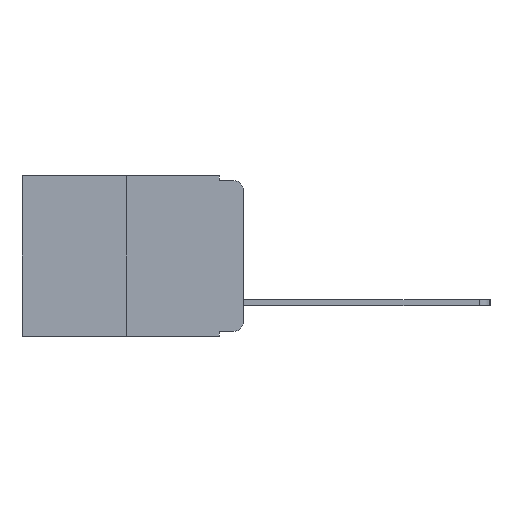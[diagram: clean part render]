
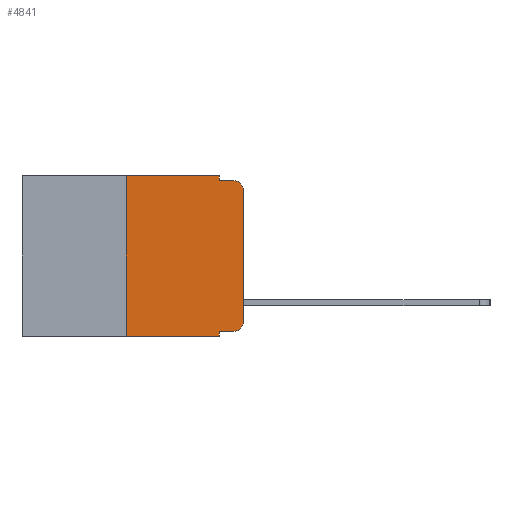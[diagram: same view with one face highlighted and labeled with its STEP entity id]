
A CAD part, left-side view. The second image highlights one B-rep face of the part: STEP entity #4841.
In plain terms, the highlighted planar face has unit normal (-1, 0, 0).
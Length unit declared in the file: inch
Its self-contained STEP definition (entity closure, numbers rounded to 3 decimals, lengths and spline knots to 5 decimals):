
#115 = ORIENTED_EDGE ( 'NONE', *, *, #9073, .F. ) ;
#141 = DIRECTION ( 'NONE',  ( 0., -1., 0. ) ) ;
#183 = CARTESIAN_POINT ( 'NONE',  ( 0., 0.02, -0.333 ) ) ;
#199 = DIRECTION ( 'NONE',  ( -1., 0., 0. ) ) ;
#259 = DIRECTION ( 'NONE',  ( 0., -1., 0. ) ) ;
#313 = VECTOR ( 'NONE', #8239, 39.37008 ) ;
#364 = VECTOR ( 'NONE', #259, 39.37008 ) ;
#525 = CARTESIAN_POINT ( 'NONE',  ( 0., 0.25, 0. ) ) ;
#972 = VECTOR ( 'NONE', #3164, 39.37008 ) ;
#1045 = VERTEX_POINT ( 'NONE', #7427 ) ;
#1091 = VERTEX_POINT ( 'NONE', #3987 ) ;
#1129 = VECTOR ( 'NONE', #141, 39.37008 ) ;
#1151 = DIRECTION ( 'NONE',  ( 0., 0., -1. ) ) ;
#1153 = LINE ( 'NONE', #5002, #7316 ) ;
#1173 = DIRECTION ( 'NONE',  ( 0., 0., 1. ) ) ;
#1389 = CARTESIAN_POINT ( 'NONE',  ( 0., 0.02, -0.313 ) ) ;
#1415 = LINE ( 'NONE', #10607, #1129 ) ;
#1475 = EDGE_CURVE ( 'NONE', #5974, #2383, #7640, .T. ) ;
#1546 = CARTESIAN_POINT ( 'NONE',  ( 0., 0.051, 0. ) ) ;
#1786 = VERTEX_POINT ( 'NONE', #6154 ) ;
#1915 = DIRECTION ( 'NONE',  ( 0., -1., 0. ) ) ;
#2142 = DIRECTION ( 'NONE',  ( 1., 0., 0. ) ) ;
#2383 = VERTEX_POINT ( 'NONE', #1546 ) ;
#2727 = CARTESIAN_POINT ( 'NONE',  ( 0., 0.051, -0.01 ) ) ;
#2735 = ORIENTED_EDGE ( 'NONE', *, *, #7925, .T. ) ;
#2810 = CARTESIAN_POINT ( 'NONE',  ( 0., 0.051, -0.01 ) ) ;
#2993 = VERTEX_POINT ( 'NONE', #4615 ) ;
#3016 = EDGE_CURVE ( 'NONE', #1786, #1045, #1415, .T. ) ;
#3032 = EDGE_CURVE ( 'NONE', #6423, #1091, #10123, .T. ) ;
#3164 = DIRECTION ( 'NONE',  ( 0., 0., 1. ) ) ;
#3453 = ORIENTED_EDGE ( 'NONE', *, *, #6531, .F. ) ;
#3987 = CARTESIAN_POINT ( 'NONE',  ( 0., 0.02, -0.01 ) ) ;
#4175 = AXIS2_PLACEMENT_3D ( 'NONE', #5494, #199, #6338 ) ;
#4245 = EDGE_CURVE ( 'NONE', #1786, #5974, #5395, .T. ) ;
#4615 = CARTESIAN_POINT ( 'NONE',  ( 0., 0., -0.313 ) ) ;
#4723 = CARTESIAN_POINT ( 'NONE',  ( 0., 0., 0. ) ) ;
#4762 = CARTESIAN_POINT ( 'NONE',  ( 0., 0.051, 0. ) ) ;
#4841 = ADVANCED_FACE ( 'NONE', ( #8622 ), #7584, .F. ) ;
#4946 = ORIENTED_EDGE ( 'NONE', *, *, #8287, .T. ) ;
#5002 = CARTESIAN_POINT ( 'NONE',  ( 0., 0.051, -0.333 ) ) ;
#5014 = EDGE_CURVE ( 'NONE', #6117, #2993, #6710, .T. ) ;
#5177 = VECTOR ( 'NONE', #1173, 39.37008 ) ;
#5386 = DIRECTION ( 'NONE',  ( 0., 0., -1. ) ) ;
#5395 = LINE ( 'NONE', #525, #972 ) ;
#5494 = CARTESIAN_POINT ( 'NONE',  ( 0., 0.02, -0.03 ) ) ;
#5552 = VECTOR ( 'NONE', #1915, 39.37008 ) ;
#5697 = AXIS2_PLACEMENT_3D ( 'NONE', #1389, #10522, #5386 ) ;
#5878 = CARTESIAN_POINT ( 'NONE',  ( 0., 0.473, 0. ) ) ;
#5974 = VERTEX_POINT ( 'NONE', #6621 ) ;
#6117 = VERTEX_POINT ( 'NONE', #183 ) ;
#6154 = CARTESIAN_POINT ( 'NONE',  ( 0., 0.25, -0.343 ) ) ;
#6241 = VERTEX_POINT ( 'NONE', #9814 ) ;
#6291 = ORIENTED_EDGE ( 'NONE', *, *, #4245, .F. ) ;
#6338 = DIRECTION ( 'NONE',  ( 0., 0., -1. ) ) ;
#6384 = VERTEX_POINT ( 'NONE', #9324 ) ;
#6423 = VERTEX_POINT ( 'NONE', #2727 ) ;
#6531 = EDGE_CURVE ( 'NONE', #2383, #6423, #9672, .T. ) ;
#6621 = CARTESIAN_POINT ( 'NONE',  ( 0., 0.25, 0. ) ) ;
#6635 = CIRCLE ( 'NONE', #4175, 0.02 ) ;
#6710 = CIRCLE ( 'NONE', #5697, 0.02 ) ;
#7316 = VECTOR ( 'NONE', #8485, 39.37008 ) ;
#7359 = VECTOR ( 'NONE', #1151, 39.37008 ) ;
#7427 = CARTESIAN_POINT ( 'NONE',  ( 0., 0.051, -0.343 ) ) ;
#7468 = LINE ( 'NONE', #4723, #5177 ) ;
#7584 = PLANE ( 'NONE',  #9954 ) ;
#7640 = LINE ( 'NONE', #8256, #364 ) ;
#7653 = ORIENTED_EDGE ( 'NONE', *, *, #5014, .T. ) ;
#7697 = EDGE_CURVE ( 'NONE', #2993, #6241, #7468, .T. ) ;
#7787 = ORIENTED_EDGE ( 'NONE', *, *, #3032, .F. ) ;
#7925 = EDGE_CURVE ( 'NONE', #6384, #6117, #1153, .T. ) ;
#7930 = EDGE_LOOP ( 'NONE', ( #8194, #4946, #7787, #3453, #10323, #6291, #11118, #115, #2735, #7653 ) ) ;
#8131 = CARTESIAN_POINT ( 'NONE',  ( 0., 0.051, 0. ) ) ;
#8194 = ORIENTED_EDGE ( 'NONE', *, *, #7697, .T. ) ;
#8239 = DIRECTION ( 'NONE',  ( 0., 0., -1. ) ) ;
#8256 = CARTESIAN_POINT ( 'NONE',  ( 0., 0.473, 0. ) ) ;
#8259 = DIRECTION ( 'NONE',  ( 0., 0., -1. ) ) ;
#8287 = EDGE_CURVE ( 'NONE', #6241, #1091, #6635, .T. ) ;
#8485 = DIRECTION ( 'NONE',  ( 0., -1., 0. ) ) ;
#8622 = FACE_OUTER_BOUND ( 'NONE', #7930, .T. ) ;
#9073 = EDGE_CURVE ( 'NONE', #6384, #1045, #9624, .T. ) ;
#9324 = CARTESIAN_POINT ( 'NONE',  ( 0., 0.051, -0.333 ) ) ;
#9624 = LINE ( 'NONE', #4762, #313 ) ;
#9672 = LINE ( 'NONE', #8131, #7359 ) ;
#9814 = CARTESIAN_POINT ( 'NONE',  ( 0., 0., -0.03 ) ) ;
#9954 = AXIS2_PLACEMENT_3D ( 'NONE', #5878, #2142, #8259 ) ;
#10123 = LINE ( 'NONE', #2810, #5552 ) ;
#10323 = ORIENTED_EDGE ( 'NONE', *, *, #1475, .F. ) ;
#10522 = DIRECTION ( 'NONE',  ( -1., 0., 0. ) ) ;
#10607 = CARTESIAN_POINT ( 'NONE',  ( 0., 0.473, -0.343 ) ) ;
#11118 = ORIENTED_EDGE ( 'NONE', *, *, #3016, .T. ) ;
